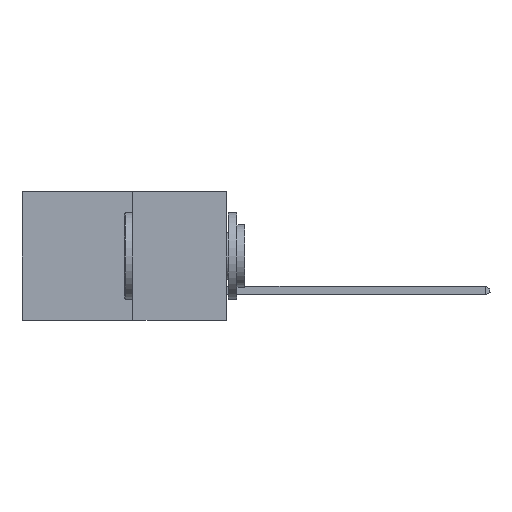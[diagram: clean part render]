
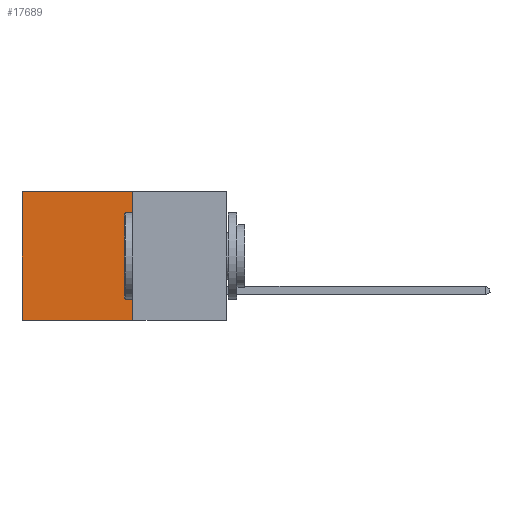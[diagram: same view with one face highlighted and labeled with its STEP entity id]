
A CAD part, left-side view. The second image highlights one B-rep face of the part: STEP entity #17689.
In plain terms, the highlighted planar face has unit normal (-1, 0, 0).
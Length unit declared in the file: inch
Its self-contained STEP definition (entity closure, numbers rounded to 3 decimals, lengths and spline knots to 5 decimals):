
#23 = VERTEX_POINT ( 'NONE', #19356 ) ;
#289 = ORIENTED_EDGE ( 'NONE', *, *, #13448, .F. ) ;
#1495 = VECTOR ( 'NONE', #13018, 39.37008 ) ;
#2076 = VECTOR ( 'NONE', #12357, 39.37008 ) ;
#2697 = LINE ( 'NONE', #21935, #2076 ) ;
#4025 = CARTESIAN_POINT ( 'NONE',  ( 0.277, 0.27, -0.37 ) ) ;
#4905 = CARTESIAN_POINT ( 'NONE',  ( 0.277, 0.27, -0.37 ) ) ;
#5724 = DIRECTION ( 'NONE',  ( 0., 1., 0. ) ) ;
#6920 = VECTOR ( 'NONE', #13743, 39.37008 ) ;
#7321 = VERTEX_POINT ( 'NONE', #8622 ) ;
#7518 = LINE ( 'NONE', #4025, #6920 ) ;
#8622 = CARTESIAN_POINT ( 'NONE',  ( 0.277, 0.59, 0. ) ) ;
#8733 = CARTESIAN_POINT ( 'NONE',  ( 0.277, 0.27, -0.37 ) ) ;
#10676 = DIRECTION ( 'NONE',  ( 0., 0., -1. ) ) ;
#11850 = ORIENTED_EDGE ( 'NONE', *, *, #18821, .T. ) ;
#12333 = EDGE_CURVE ( 'NONE', #7321, #23, #22132, .T. ) ;
#12357 = DIRECTION ( 'NONE',  ( 0., 1., 0. ) ) ;
#12462 = VECTOR ( 'NONE', #5724, 39.37008 ) ;
#13018 = DIRECTION ( 'NONE',  ( 0., 0., -1. ) ) ;
#13393 = ORIENTED_EDGE ( 'NONE', *, *, #13466, .F. ) ;
#13448 = EDGE_CURVE ( 'NONE', #23241, #17096, #7518, .T. ) ;
#13466 = EDGE_CURVE ( 'NONE', #17096, #23, #17581, .T. ) ;
#13743 = DIRECTION ( 'NONE',  ( 0., 0., -1. ) ) ;
#13823 = EDGE_LOOP ( 'NONE', ( #24981, #13393, #289, #11850 ) ) ;
#14520 = PLANE ( 'NONE',  #15278 ) ;
#15278 = AXIS2_PLACEMENT_3D ( 'NONE', #8733, #22227, #10676 ) ;
#17096 = VERTEX_POINT ( 'NONE', #4905 ) ;
#17581 = LINE ( 'NONE', #21111, #12462 ) ;
#17689 = ADVANCED_FACE ( 'NONE', ( #23058 ), #14520, .F. ) ;
#18821 = EDGE_CURVE ( 'NONE', #23241, #7321, #2697, .T. ) ;
#19356 = CARTESIAN_POINT ( 'NONE',  ( 0.277, 0.59, -0.37 ) ) ;
#20644 = CARTESIAN_POINT ( 'NONE',  ( 0.277, 0.27, 0. ) ) ;
#21111 = CARTESIAN_POINT ( 'NONE',  ( 0.277, 0.27, -0.37 ) ) ;
#21935 = CARTESIAN_POINT ( 'NONE',  ( 0.277, 0.27, 0. ) ) ;
#22132 = LINE ( 'NONE', #22582, #1495 ) ;
#22227 = DIRECTION ( 'NONE',  ( 1., 0., 0. ) ) ;
#22582 = CARTESIAN_POINT ( 'NONE',  ( 0.277, 0.59, -0.37 ) ) ;
#23058 = FACE_OUTER_BOUND ( 'NONE', #13823, .T. ) ;
#23241 = VERTEX_POINT ( 'NONE', #20644 ) ;
#24981 = ORIENTED_EDGE ( 'NONE', *, *, #12333, .T. ) ;
